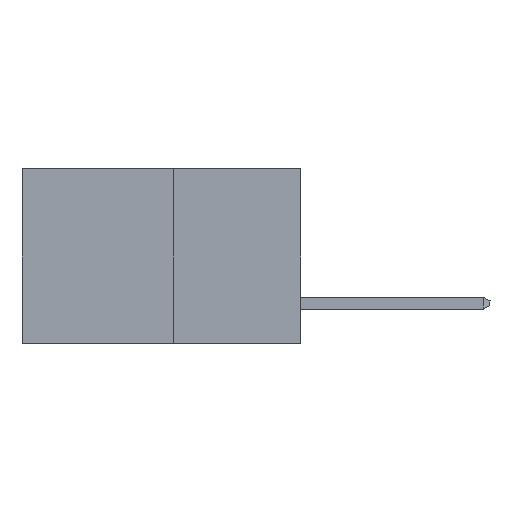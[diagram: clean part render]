
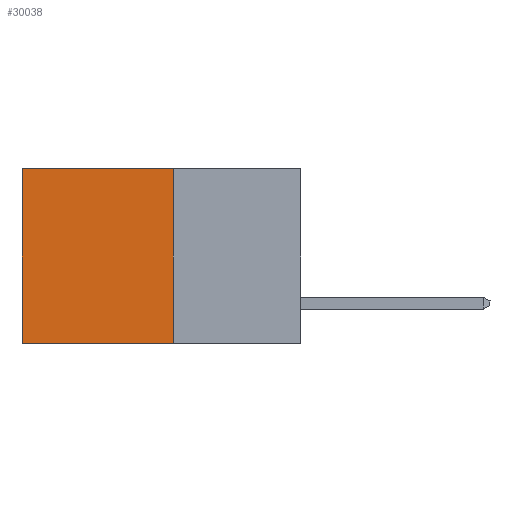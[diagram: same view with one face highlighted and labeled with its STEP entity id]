
A CAD part, left-side view. The second image highlights one B-rep face of the part: STEP entity #30038.
In plain terms, the highlighted planar face has unit normal (-1, 0, 0).
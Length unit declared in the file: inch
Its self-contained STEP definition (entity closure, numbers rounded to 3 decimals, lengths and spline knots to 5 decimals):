
#738 = LINE ( 'NONE', #28471, #7787 ) ;
#3858 = LINE ( 'NONE', #5192, #15344 ) ;
#5192 = CARTESIAN_POINT ( 'NONE',  ( 0.277, 0.27, -0.37 ) ) ;
#5877 = VECTOR ( 'NONE', #13070, 39.37008 ) ;
#7630 = EDGE_CURVE ( 'NONE', #28328, #12785, #738, .T. ) ;
#7787 = VECTOR ( 'NONE', #20328, 39.37008 ) ;
#8857 = EDGE_LOOP ( 'NONE', ( #15771, #18270, #30077, #11664 ) ) ;
#9491 = VERTEX_POINT ( 'NONE', #11025 ) ;
#9638 = LINE ( 'NONE', #15632, #15815 ) ;
#9984 = DIRECTION ( 'NONE',  ( 0., 0., -1. ) ) ;
#11025 = CARTESIAN_POINT ( 'NONE',  ( 0.277, 0.27, -0.37 ) ) ;
#11664 = ORIENTED_EDGE ( 'NONE', *, *, #32518, .T. ) ;
#12785 = VERTEX_POINT ( 'NONE', #21292 ) ;
#12844 = LINE ( 'NONE', #28655, #5877 ) ;
#13070 = DIRECTION ( 'NONE',  ( 0., 1., 0. ) ) ;
#15344 = VECTOR ( 'NONE', #31393, 39.37008 ) ;
#15632 = CARTESIAN_POINT ( 'NONE',  ( 0.277, 0.27, -0.37 ) ) ;
#15716 = CARTESIAN_POINT ( 'NONE',  ( 0.277, 0.59, 0. ) ) ;
#15771 = ORIENTED_EDGE ( 'NONE', *, *, #7630, .T. ) ;
#15815 = VECTOR ( 'NONE', #18307, 39.37008 ) ;
#18270 = ORIENTED_EDGE ( 'NONE', *, *, #27678, .F. ) ;
#18307 = DIRECTION ( 'NONE',  ( 0., 0., -1. ) ) ;
#19981 = CARTESIAN_POINT ( 'NONE',  ( 0.277, 0.27, 0. ) ) ;
#20328 = DIRECTION ( 'NONE',  ( 0., 0., -1. ) ) ;
#20432 = CARTESIAN_POINT ( 'NONE',  ( 0.277, 0.27, -0.37 ) ) ;
#20506 = AXIS2_PLACEMENT_3D ( 'NONE', #20432, #25689, #9984 ) ;
#21292 = CARTESIAN_POINT ( 'NONE',  ( 0.277, 0.59, -0.37 ) ) ;
#21560 = EDGE_CURVE ( 'NONE', #28094, #9491, #9638, .T. ) ;
#23055 = PLANE ( 'NONE',  #20506 ) ;
#25689 = DIRECTION ( 'NONE',  ( 1., 0., 0. ) ) ;
#27678 = EDGE_CURVE ( 'NONE', #9491, #12785, #3858, .T. ) ;
#28094 = VERTEX_POINT ( 'NONE', #19981 ) ;
#28190 = FACE_OUTER_BOUND ( 'NONE', #8857, .T. ) ;
#28328 = VERTEX_POINT ( 'NONE', #15716 ) ;
#28471 = CARTESIAN_POINT ( 'NONE',  ( 0.277, 0.59, -0.37 ) ) ;
#28655 = CARTESIAN_POINT ( 'NONE',  ( 0.277, 0.27, 0. ) ) ;
#30038 = ADVANCED_FACE ( 'NONE', ( #28190 ), #23055, .F. ) ;
#30077 = ORIENTED_EDGE ( 'NONE', *, *, #21560, .F. ) ;
#31393 = DIRECTION ( 'NONE',  ( 0., 1., 0. ) ) ;
#32518 = EDGE_CURVE ( 'NONE', #28094, #28328, #12844, .T. ) ;
